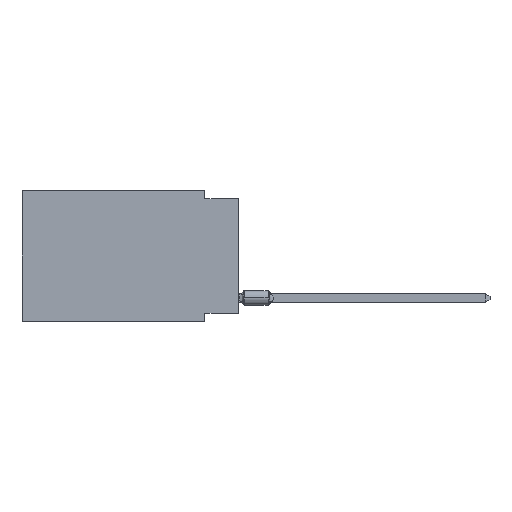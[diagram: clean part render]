
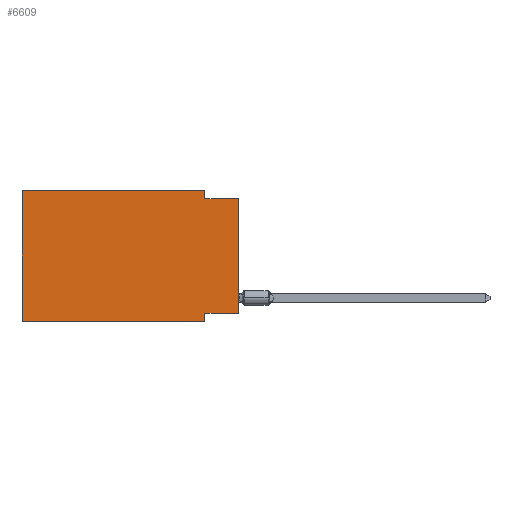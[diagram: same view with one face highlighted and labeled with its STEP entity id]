
A CAD part, left-side view. The second image highlights one B-rep face of the part: STEP entity #6609.
In plain terms, the highlighted planar face has unit normal (-1, 0, 0).
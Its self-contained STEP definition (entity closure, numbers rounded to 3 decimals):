
#5 = DIRECTION ( 'NONE',  ( 0., 0., 1. ) ) ;
#75 = CARTESIAN_POINT ( 'NONE',  ( 0., 0., 0. ) ) ;
#294 = DIRECTION ( 'NONE',  ( 0., 0., -1. ) ) ;
#307 = ORIENTED_EDGE ( 'NONE', *, *, #3843, .F. ) ;
#947 = CARTESIAN_POINT ( 'NONE',  ( 0., 16.383, -9.906 ) ) ;
#1638 = CARTESIAN_POINT ( 'NONE',  ( 0., 16.383, 0. ) ) ;
#1893 = DIRECTION ( 'NONE',  ( 0., -1., 0. ) ) ;
#1923 = VERTEX_POINT ( 'NONE', #7902 ) ;
#2210 = CARTESIAN_POINT ( 'NONE',  ( 0., 16.383, -9.906 ) ) ;
#2518 = VERTEX_POINT ( 'NONE', #6399 ) ;
#2553 = EDGE_CURVE ( 'NONE', #8860, #2518, #3308, .T. ) ;
#3039 = AXIS2_PLACEMENT_3D ( 'NONE', #9308, #3947, #294 ) ;
#3297 = VECTOR ( 'NONE', #11699, 1000. ) ;
#3308 = LINE ( 'NONE', #9823, #5985 ) ;
#3348 = ORIENTED_EDGE ( 'NONE', *, *, #10957, .T. ) ;
#3628 = DIRECTION ( 'NONE',  ( 0., 0., -1. ) ) ;
#3843 = EDGE_CURVE ( 'NONE', #10195, #5155, #7668, .T. ) ;
#3852 = ORIENTED_EDGE ( 'NONE', *, *, #6550, .F. ) ;
#3873 = LINE ( 'NONE', #1638, #6255 ) ;
#3947 = DIRECTION ( 'NONE',  ( 1., 0., 0. ) ) ;
#3950 = ORIENTED_EDGE ( 'NONE', *, *, #13230, .F. ) ;
#4316 = DIRECTION ( 'NONE',  ( 0., 0., -1. ) ) ;
#4451 = DIRECTION ( 'NONE',  ( 0., 1., 0. ) ) ;
#4622 = LINE ( 'NONE', #13426, #11646 ) ;
#4957 = CARTESIAN_POINT ( 'NONE',  ( 0., 2.54, 0. ) ) ;
#5108 = DIRECTION ( 'NONE',  ( 0., -1., 0. ) ) ;
#5155 = VERTEX_POINT ( 'NONE', #6962 ) ;
#5762 = EDGE_CURVE ( 'NONE', #5155, #1923, #4622, .T. ) ;
#5985 = VECTOR ( 'NONE', #4316, 1000. ) ;
#6011 = PLANE ( 'NONE',  #3039 ) ;
#6190 = CARTESIAN_POINT ( 'NONE',  ( 0., 16.383, 0. ) ) ;
#6253 = LINE ( 'NONE', #7524, #12449 ) ;
#6255 = VECTOR ( 'NONE', #9383, 1000. ) ;
#6256 = LINE ( 'NONE', #947, #3297 ) ;
#6399 = CARTESIAN_POINT ( 'NONE',  ( 0., 2.54, -0.635 ) ) ;
#6550 = EDGE_CURVE ( 'NONE', #9508, #13959, #3873, .T. ) ;
#6609 = ADVANCED_FACE ( 'NONE', ( #12534 ), #6011, .F. ) ;
#6650 = LINE ( 'NONE', #75, #6675 ) ;
#6675 = VECTOR ( 'NONE', #5, 1000. ) ;
#6962 = CARTESIAN_POINT ( 'NONE',  ( 0., 2.54, -9.271 ) ) ;
#7407 = LINE ( 'NONE', #6190, #13921 ) ;
#7524 = CARTESIAN_POINT ( 'NONE',  ( 0., 0., -0.635 ) ) ;
#7668 = LINE ( 'NONE', #12047, #7817 ) ;
#7809 = EDGE_CURVE ( 'NONE', #2518, #9473, #6253, .T. ) ;
#7817 = VECTOR ( 'NONE', #4451, 1000. ) ;
#7902 = CARTESIAN_POINT ( 'NONE',  ( 0., 2.54, -9.906 ) ) ;
#7906 = ORIENTED_EDGE ( 'NONE', *, *, #2553, .F. ) ;
#8239 = CARTESIAN_POINT ( 'NONE',  ( 0., 16.383, 0. ) ) ;
#8860 = VERTEX_POINT ( 'NONE', #4957 ) ;
#8946 = EDGE_CURVE ( 'NONE', #9508, #1923, #6256, .T. ) ;
#9308 = CARTESIAN_POINT ( 'NONE',  ( 0., 16.383, 0. ) ) ;
#9383 = DIRECTION ( 'NONE',  ( 0., 0., 1. ) ) ;
#9473 = VERTEX_POINT ( 'NONE', #12164 ) ;
#9508 = VERTEX_POINT ( 'NONE', #2210 ) ;
#9823 = CARTESIAN_POINT ( 'NONE',  ( 0., 2.54, 0. ) ) ;
#10195 = VERTEX_POINT ( 'NONE', #10869 ) ;
#10256 = ORIENTED_EDGE ( 'NONE', *, *, #5762, .F. ) ;
#10421 = EDGE_LOOP ( 'NONE', ( #3348, #11712, #7906, #3950, #3852, #11394, #10256, #307 ) ) ;
#10869 = CARTESIAN_POINT ( 'NONE',  ( 0., 0., -9.271 ) ) ;
#10957 = EDGE_CURVE ( 'NONE', #10195, #9473, #6650, .T. ) ;
#11394 = ORIENTED_EDGE ( 'NONE', *, *, #8946, .T. ) ;
#11646 = VECTOR ( 'NONE', #3628, 1000. ) ;
#11699 = DIRECTION ( 'NONE',  ( 0., -1., 0. ) ) ;
#11712 = ORIENTED_EDGE ( 'NONE', *, *, #7809, .F. ) ;
#12047 = CARTESIAN_POINT ( 'NONE',  ( 0., 0., -9.271 ) ) ;
#12164 = CARTESIAN_POINT ( 'NONE',  ( 0., 0., -0.635 ) ) ;
#12449 = VECTOR ( 'NONE', #5108, 1000. ) ;
#12534 = FACE_OUTER_BOUND ( 'NONE', #10421, .T. ) ;
#13230 = EDGE_CURVE ( 'NONE', #13959, #8860, #7407, .T. ) ;
#13426 = CARTESIAN_POINT ( 'NONE',  ( 0., 2.54, -9.906 ) ) ;
#13921 = VECTOR ( 'NONE', #1893, 1000. ) ;
#13959 = VERTEX_POINT ( 'NONE', #8239 ) ;
